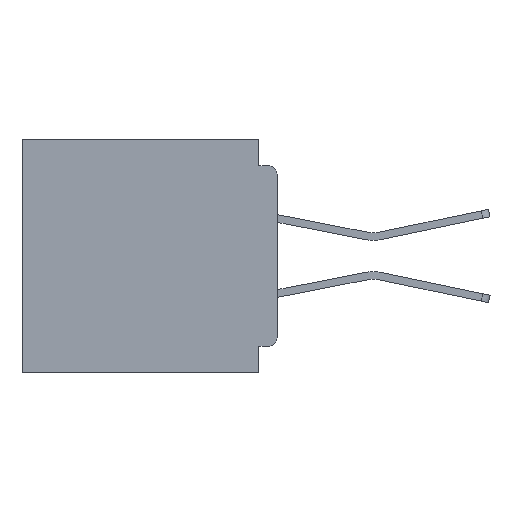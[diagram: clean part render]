
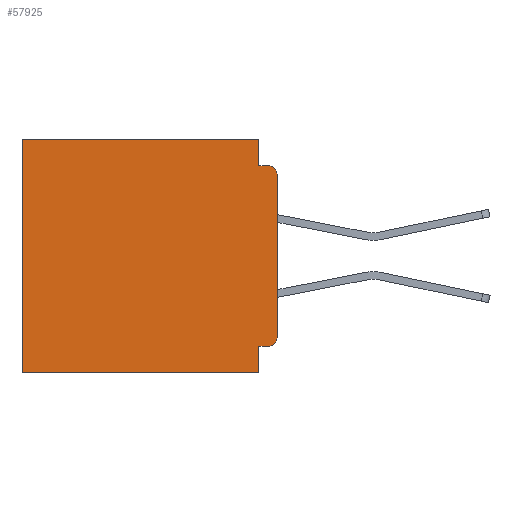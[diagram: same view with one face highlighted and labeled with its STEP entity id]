
A CAD part, left-side view. The second image highlights one B-rep face of the part: STEP entity #57925.
In plain terms, the highlighted planar face has unit normal (-1, 0, 0).
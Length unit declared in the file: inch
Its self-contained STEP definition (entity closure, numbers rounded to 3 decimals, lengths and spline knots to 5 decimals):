
#309 = LINE ( 'NONE', #49234, #34009 ) ;
#1743 = AXIS2_PLACEMENT_3D ( 'NONE', #6772, #38838, #11419 ) ;
#1819 = DIRECTION ( 'NONE',  ( 1., 0., 0. ) ) ;
#1943 = VERTEX_POINT ( 'NONE', #23023 ) ;
#2258 = EDGE_CURVE ( 'NONE', #11179, #16483, #58632, .T. ) ;
#2467 = VECTOR ( 'NONE', #44687, 39.37008 ) ;
#2836 = VERTEX_POINT ( 'NONE', #45645 ) ;
#2870 = LINE ( 'NONE', #52360, #21518 ) ;
#2925 = CARTESIAN_POINT ( 'NONE',  ( 0.3, 0.437, 0. ) ) ;
#4129 = CARTESIAN_POINT ( 'NONE',  ( 0.3, 0.031, 0. ) ) ;
#4619 = AXIS2_PLACEMENT_3D ( 'NONE', #6211, #1819, #33885 ) ;
#6211 = CARTESIAN_POINT ( 'NONE',  ( 0.3, 0., -0.4 ) ) ;
#6772 = CARTESIAN_POINT ( 'NONE',  ( 0.3, 0.015, -0.34 ) ) ;
#8261 = CIRCLE ( 'NONE', #53781, 0.015 ) ;
#9079 = EDGE_CURVE ( 'NONE', #11179, #41062, #8261, .T. ) ;
#9340 = CARTESIAN_POINT ( 'NONE',  ( 0.3, 0., -0.045 ) ) ;
#9455 = EDGE_CURVE ( 'NONE', #27624, #29414, #309, .T. ) ;
#11179 = VERTEX_POINT ( 'NONE', #39649 ) ;
#11419 = DIRECTION ( 'NONE',  ( 0., 0., -1. ) ) ;
#12389 = CARTESIAN_POINT ( 'NONE',  ( 0.3, 0., -0.34 ) ) ;
#12646 = VECTOR ( 'NONE', #36171, 39.37008 ) ;
#13009 = DIRECTION ( 'NONE',  ( 0., 1., 0. ) ) ;
#13584 = CARTESIAN_POINT ( 'NONE',  ( 0.3, 0.015, -0.045 ) ) ;
#14626 = DIRECTION ( 'NONE',  ( -1., 0., 0. ) ) ;
#14645 = CARTESIAN_POINT ( 'NONE',  ( 0.3, 0.437, -0.4 ) ) ;
#15646 = VECTOR ( 'NONE', #13009, 39.37008 ) ;
#16483 = VERTEX_POINT ( 'NONE', #12389 ) ;
#20386 = DIRECTION ( 'NONE',  ( 0., 1., 0. ) ) ;
#21518 = VECTOR ( 'NONE', #20386, 39.37008 ) ;
#21872 = CARTESIAN_POINT ( 'NONE',  ( 0.3, 0.437, -0.4 ) ) ;
#21930 = EDGE_CURVE ( 'NONE', #29151, #48392, #2870, .T. ) ;
#22697 = DIRECTION ( 'NONE',  ( 0., 0., -1. ) ) ;
#22863 = VECTOR ( 'NONE', #59135, 39.37008 ) ;
#23023 = CARTESIAN_POINT ( 'NONE',  ( 0.3, 0.015, -0.355 ) ) ;
#24315 = LINE ( 'NONE', #49963, #22863 ) ;
#26579 = CARTESIAN_POINT ( 'NONE',  ( 0.3, 0.031, 0. ) ) ;
#26646 = VECTOR ( 'NONE', #45970, 39.37008 ) ;
#27624 = VERTEX_POINT ( 'NONE', #54054 ) ;
#27867 = LINE ( 'NONE', #40443, #15646 ) ;
#28327 = EDGE_CURVE ( 'NONE', #46028, #27624, #24315, .T. ) ;
#29151 = VERTEX_POINT ( 'NONE', #26579 ) ;
#29414 = VERTEX_POINT ( 'NONE', #14645 ) ;
#30520 = EDGE_CURVE ( 'NONE', #29151, #2836, #58441, .T. ) ;
#31059 = DIRECTION ( 'NONE',  ( 0., 1., 0. ) ) ;
#31571 = EDGE_CURVE ( 'NONE', #48392, #29414, #39023, .T. ) ;
#32811 = ORIENTED_EDGE ( 'NONE', *, *, #55019, .F. ) ;
#33287 = ORIENTED_EDGE ( 'NONE', *, *, #40330, .F. ) ;
#33885 = DIRECTION ( 'NONE',  ( 0., 0., -1. ) ) ;
#34009 = VECTOR ( 'NONE', #31059, 39.37008 ) ;
#34248 = ORIENTED_EDGE ( 'NONE', *, *, #42678, .T. ) ;
#36171 = DIRECTION ( 'NONE',  ( 0., 0., -1. ) ) ;
#38838 = DIRECTION ( 'NONE',  ( -1., 0., 0. ) ) ;
#39023 = LINE ( 'NONE', #21872, #2467 ) ;
#39649 = CARTESIAN_POINT ( 'NONE',  ( 0.3, 0., -0.06 ) ) ;
#39829 = CARTESIAN_POINT ( 'NONE',  ( 0.3, 0., -0.4 ) ) ;
#40128 = EDGE_LOOP ( 'NONE', ( #43868, #41323, #32811, #48052, #40684, #40471, #45865, #42214, #33287, #34248 ) ) ;
#40330 = EDGE_CURVE ( 'NONE', #1943, #46028, #27867, .T. ) ;
#40443 = CARTESIAN_POINT ( 'NONE',  ( 0.3, 0., -0.355 ) ) ;
#40471 = ORIENTED_EDGE ( 'NONE', *, *, #31571, .T. ) ;
#40684 = ORIENTED_EDGE ( 'NONE', *, *, #21930, .T. ) ;
#41062 = VERTEX_POINT ( 'NONE', #13584 ) ;
#41323 = ORIENTED_EDGE ( 'NONE', *, *, #9079, .T. ) ;
#42081 = CARTESIAN_POINT ( 'NONE',  ( 0.3, 0.015, -0.06 ) ) ;
#42214 = ORIENTED_EDGE ( 'NONE', *, *, #28327, .F. ) ;
#42678 = EDGE_CURVE ( 'NONE', #1943, #16483, #56229, .T. ) ;
#43868 = ORIENTED_EDGE ( 'NONE', *, *, #2258, .F. ) ;
#44687 = DIRECTION ( 'NONE',  ( 0., 0., -1. ) ) ;
#45645 = CARTESIAN_POINT ( 'NONE',  ( 0.3, 0.031, -0.045 ) ) ;
#45865 = ORIENTED_EDGE ( 'NONE', *, *, #9455, .F. ) ;
#45970 = DIRECTION ( 'NONE',  ( 0., -1., 0. ) ) ;
#46028 = VERTEX_POINT ( 'NONE', #53698 ) ;
#46680 = DIRECTION ( 'NONE',  ( 0., 0., -1. ) ) ;
#47304 = VECTOR ( 'NONE', #22697, 39.37008 ) ;
#48052 = ORIENTED_EDGE ( 'NONE', *, *, #30520, .F. ) ;
#48392 = VERTEX_POINT ( 'NONE', #2925 ) ;
#49234 = CARTESIAN_POINT ( 'NONE',  ( 0.3, 0., -0.4 ) ) ;
#49963 = CARTESIAN_POINT ( 'NONE',  ( 0.3, 0.031, -0.4 ) ) ;
#50935 = LINE ( 'NONE', #9340, #26646 ) ;
#52360 = CARTESIAN_POINT ( 'NONE',  ( 0.3, 0., 0. ) ) ;
#53698 = CARTESIAN_POINT ( 'NONE',  ( 0.3, 0.031, -0.355 ) ) ;
#53781 = AXIS2_PLACEMENT_3D ( 'NONE', #42081, #14626, #46680 ) ;
#54054 = CARTESIAN_POINT ( 'NONE',  ( 0.3, 0.031, -0.4 ) ) ;
#55019 = EDGE_CURVE ( 'NONE', #2836, #41062, #50935, .T. ) ;
#55716 = FACE_OUTER_BOUND ( 'NONE', #40128, .T. ) ;
#56229 = CIRCLE ( 'NONE', #1743, 0.015 ) ;
#56651 = PLANE ( 'NONE',  #4619 ) ;
#57925 = ADVANCED_FACE ( 'NONE', ( #55716 ), #56651, .F. ) ;
#58441 = LINE ( 'NONE', #4129, #12646 ) ;
#58632 = LINE ( 'NONE', #39829, #47304 ) ;
#59135 = DIRECTION ( 'NONE',  ( 0., 0., -1. ) ) ;
